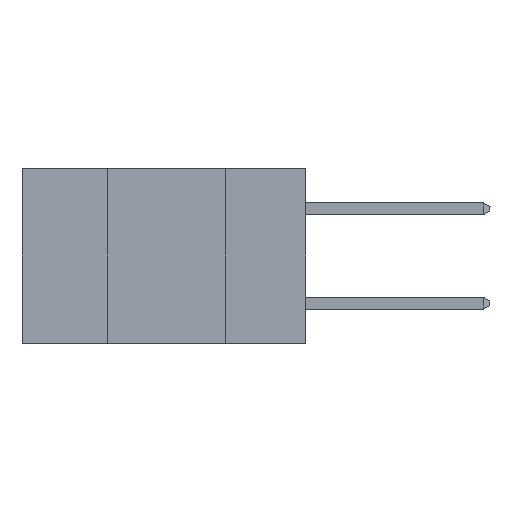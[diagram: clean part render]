
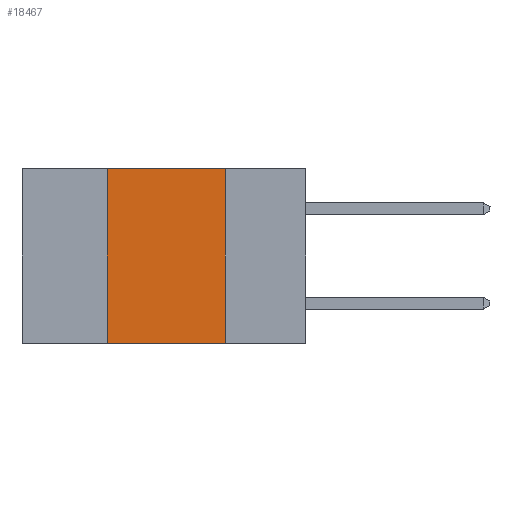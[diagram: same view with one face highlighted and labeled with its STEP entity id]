
A CAD part, left-side view. The second image highlights one B-rep face of the part: STEP entity #18467.
In plain terms, the highlighted planar face has unit normal (-1, 0, 0).
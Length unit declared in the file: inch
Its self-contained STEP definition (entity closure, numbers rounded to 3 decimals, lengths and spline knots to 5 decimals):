
#2122 = ORIENTED_EDGE ( 'NONE', *, *, #30137, .F. ) ;
#2646 = VECTOR ( 'NONE', #7487, 39.37008 ) ;
#5979 = VERTEX_POINT ( 'NONE', #25776 ) ;
#6019 = DIRECTION ( 'NONE',  ( 0., 0., 1. ) ) ;
#6164 = VERTEX_POINT ( 'NONE', #18864 ) ;
#7487 = DIRECTION ( 'NONE',  ( 0., -1., 0. ) ) ;
#7646 = VECTOR ( 'NONE', #19489, 39.37008 ) ;
#8430 = LINE ( 'NONE', #16997, #7646 ) ;
#9341 = DIRECTION ( 'NONE',  ( 0., 0., -1. ) ) ;
#12199 = CARTESIAN_POINT ( 'NONE',  ( 0., 0.17, 0. ) ) ;
#12584 = AXIS2_PLACEMENT_3D ( 'NONE', #29367, #24446, #9341 ) ;
#14046 = LINE ( 'NONE', #20171, #19914 ) ;
#14521 = ORIENTED_EDGE ( 'NONE', *, *, #19663, .F. ) ;
#15299 = EDGE_LOOP ( 'NONE', ( #2122, #28656, #14521, #32523 ) ) ;
#16997 = CARTESIAN_POINT ( 'NONE',  ( 0., 0.17, 0. ) ) ;
#18467 = ADVANCED_FACE ( 'NONE', ( #21376 ), #31838, .F. ) ;
#18864 = CARTESIAN_POINT ( 'NONE',  ( 0., 0.17, -0.37 ) ) ;
#19489 = DIRECTION ( 'NONE',  ( 0., 0., -1. ) ) ;
#19663 = EDGE_CURVE ( 'NONE', #5979, #21573, #31063, .T. ) ;
#19822 = CARTESIAN_POINT ( 'NONE',  ( 0., 0.6, -0.37 ) ) ;
#19914 = VECTOR ( 'NONE', #32627, 39.37008 ) ;
#20032 = EDGE_CURVE ( 'NONE', #5979, #6164, #22893, .T. ) ;
#20171 = CARTESIAN_POINT ( 'NONE',  ( 0., 0.6, 0. ) ) ;
#21376 = FACE_OUTER_BOUND ( 'NONE', #15299, .T. ) ;
#21573 = VERTEX_POINT ( 'NONE', #28546 ) ;
#22893 = LINE ( 'NONE', #19822, #2646 ) ;
#23210 = VERTEX_POINT ( 'NONE', #12199 ) ;
#23626 = VECTOR ( 'NONE', #6019, 39.37008 ) ;
#24073 = EDGE_CURVE ( 'NONE', #21573, #23210, #14046, .T. ) ;
#24446 = DIRECTION ( 'NONE',  ( 1., 0., 0. ) ) ;
#25776 = CARTESIAN_POINT ( 'NONE',  ( 0., 0.42, -0.37 ) ) ;
#26118 = CARTESIAN_POINT ( 'NONE',  ( 0., 0.42, 0. ) ) ;
#28546 = CARTESIAN_POINT ( 'NONE',  ( 0., 0.42, 0. ) ) ;
#28656 = ORIENTED_EDGE ( 'NONE', *, *, #24073, .F. ) ;
#29367 = CARTESIAN_POINT ( 'NONE',  ( 0., 0.6, 0. ) ) ;
#30137 = EDGE_CURVE ( 'NONE', #23210, #6164, #8430, .T. ) ;
#31063 = LINE ( 'NONE', #26118, #23626 ) ;
#31838 = PLANE ( 'NONE',  #12584 ) ;
#32523 = ORIENTED_EDGE ( 'NONE', *, *, #20032, .T. ) ;
#32627 = DIRECTION ( 'NONE',  ( 0., -1., 0. ) ) ;
